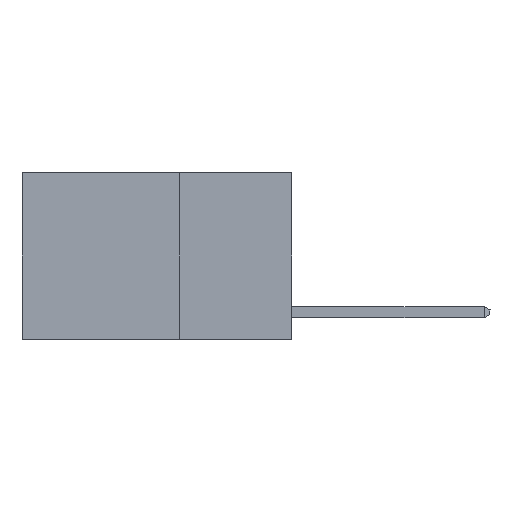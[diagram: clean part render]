
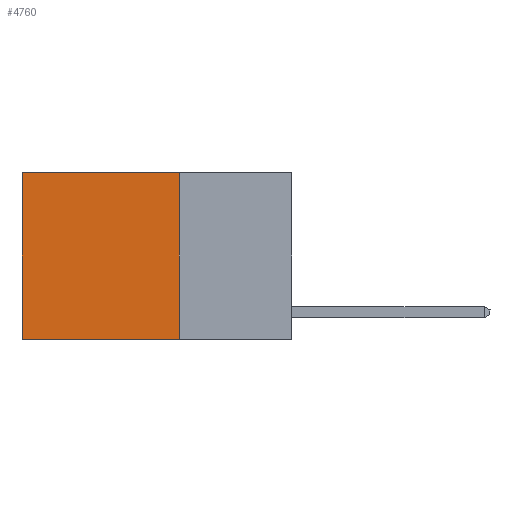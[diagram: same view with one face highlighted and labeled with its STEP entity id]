
A CAD part, left-side view. The second image highlights one B-rep face of the part: STEP entity #4760.
In plain terms, the highlighted planar face has unit normal (-1, 0, 0).
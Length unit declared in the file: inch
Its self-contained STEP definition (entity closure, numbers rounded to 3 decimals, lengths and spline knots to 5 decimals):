
#369 = FACE_OUTER_BOUND ( 'NONE', #12064, .T. ) ;
#510 = LINE ( 'NONE', #11228, #13731 ) ;
#552 = VERTEX_POINT ( 'NONE', #16919 ) ;
#1369 = VECTOR ( 'NONE', #2717, 39.37008 ) ;
#1599 = LINE ( 'NONE', #5689, #1369 ) ;
#2159 = VERTEX_POINT ( 'NONE', #4758 ) ;
#2202 = VERTEX_POINT ( 'NONE', #6164 ) ;
#2603 = VECTOR ( 'NONE', #13154, 39.37008 ) ;
#2638 = DIRECTION ( 'NONE',  ( 0., 0., -1. ) ) ;
#2717 = DIRECTION ( 'NONE',  ( 0., 1., 0. ) ) ;
#2831 = AXIS2_PLACEMENT_3D ( 'NONE', #8844, #11727, #11668 ) ;
#3258 = CARTESIAN_POINT ( 'NONE',  ( 0.2625, 0.6, 0. ) ) ;
#3344 = PLANE ( 'NONE',  #2831 ) ;
#3424 = CARTESIAN_POINT ( 'NONE',  ( 0.2625, 0.6, -0.37 ) ) ;
#3446 = LINE ( 'NONE', #15692, #14853 ) ;
#4053 = DIRECTION ( 'NONE',  ( 0., 1., 0. ) ) ;
#4758 = CARTESIAN_POINT ( 'NONE',  ( 0.2625, 0.25, -0.37 ) ) ;
#4760 = ADVANCED_FACE ( 'NONE', ( #369 ), #3344, .F. ) ;
#5689 = CARTESIAN_POINT ( 'NONE',  ( 0.2625, 0.25, -0.37 ) ) ;
#6164 = CARTESIAN_POINT ( 'NONE',  ( 0.2625, 0.6, 0. ) ) ;
#6547 = EDGE_CURVE ( 'NONE', #552, #2159, #510, .T. ) ;
#8844 = CARTESIAN_POINT ( 'NONE',  ( 0.2625, 0.25, 0. ) ) ;
#11133 = LINE ( 'NONE', #3258, #2603 ) ;
#11228 = CARTESIAN_POINT ( 'NONE',  ( 0.2625, 0.25, 0. ) ) ;
#11356 = ORIENTED_EDGE ( 'NONE', *, *, #12650, .T. ) ;
#11668 = DIRECTION ( 'NONE',  ( 0., 0., -1. ) ) ;
#11727 = DIRECTION ( 'NONE',  ( 1., 0., 0. ) ) ;
#11815 = EDGE_CURVE ( 'NONE', #2159, #14369, #1599, .T. ) ;
#12064 = EDGE_LOOP ( 'NONE', ( #11356, #14058, #18010, #13958 ) ) ;
#12650 = EDGE_CURVE ( 'NONE', #2202, #14369, #11133, .T. ) ;
#13154 = DIRECTION ( 'NONE',  ( 0., 0., -1. ) ) ;
#13731 = VECTOR ( 'NONE', #2638, 39.37008 ) ;
#13958 = ORIENTED_EDGE ( 'NONE', *, *, #16622, .T. ) ;
#14058 = ORIENTED_EDGE ( 'NONE', *, *, #11815, .F. ) ;
#14369 = VERTEX_POINT ( 'NONE', #3424 ) ;
#14853 = VECTOR ( 'NONE', #4053, 39.37008 ) ;
#15692 = CARTESIAN_POINT ( 'NONE',  ( 0.2625, 0.25, 0. ) ) ;
#16622 = EDGE_CURVE ( 'NONE', #552, #2202, #3446, .T. ) ;
#16919 = CARTESIAN_POINT ( 'NONE',  ( 0.2625, 0.25, 0. ) ) ;
#18010 = ORIENTED_EDGE ( 'NONE', *, *, #6547, .F. ) ;
